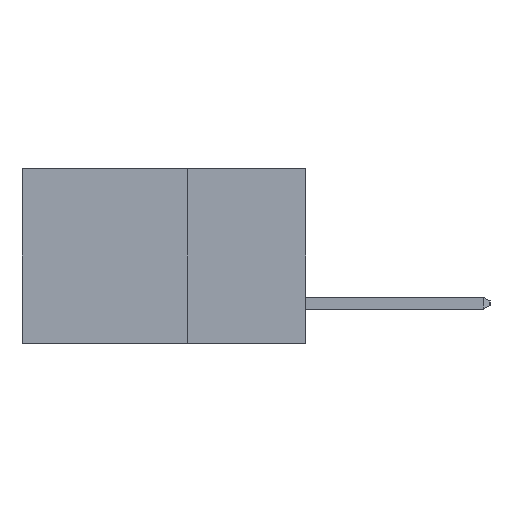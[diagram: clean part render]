
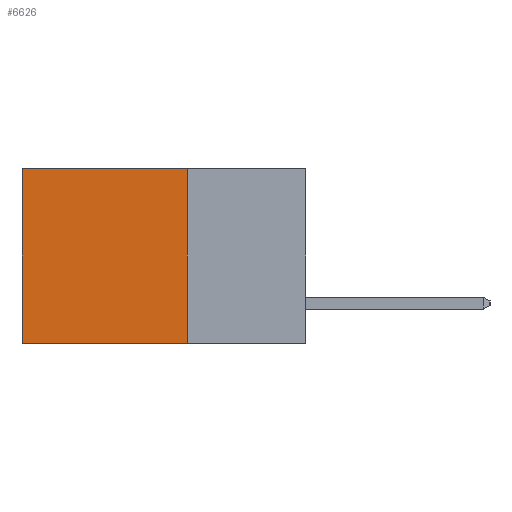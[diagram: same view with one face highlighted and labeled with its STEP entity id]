
A CAD part, left-side view. The second image highlights one B-rep face of the part: STEP entity #6626.
In plain terms, the highlighted planar face has unit normal (-1, 0, 0).
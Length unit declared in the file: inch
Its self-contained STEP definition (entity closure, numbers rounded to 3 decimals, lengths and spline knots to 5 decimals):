
#34 = CARTESIAN_POINT ( 'NONE',  ( 0.298, 0.25, 0. ) ) ;
#681 = VERTEX_POINT ( 'NONE', #8977 ) ;
#682 = EDGE_CURVE ( 'NONE', #681, #2729, #7356, .T. ) ;
#875 = CARTESIAN_POINT ( 'NONE',  ( 0.298, 0.25, 0. ) ) ;
#1124 = VECTOR ( 'NONE', #9426, 39.37008 ) ;
#1205 = DIRECTION ( 'NONE',  ( 0., 0., -1. ) ) ;
#1342 = LINE ( 'NONE', #8566, #5639 ) ;
#1620 = ORIENTED_EDGE ( 'NONE', *, *, #7671, .F. ) ;
#2339 = CARTESIAN_POINT ( 'NONE',  ( 0.298, 0.6, -0.37 ) ) ;
#2486 = VERTEX_POINT ( 'NONE', #10119 ) ;
#2727 = ORIENTED_EDGE ( 'NONE', *, *, #9683, .T. ) ;
#2729 = VERTEX_POINT ( 'NONE', #3269 ) ;
#2986 = EDGE_LOOP ( 'NONE', ( #2727, #3515, #1620, #4265 ) ) ;
#3269 = CARTESIAN_POINT ( 'NONE',  ( 0.298, 0.6, 0. ) ) ;
#3286 = LINE ( 'NONE', #7079, #1124 ) ;
#3515 = ORIENTED_EDGE ( 'NONE', *, *, #4010, .F. ) ;
#3601 = DIRECTION ( 'NONE',  ( 0., 1., 0. ) ) ;
#4010 = EDGE_CURVE ( 'NONE', #2486, #9549, #1342, .T. ) ;
#4142 = DIRECTION ( 'NONE',  ( 1., 0., 0. ) ) ;
#4265 = ORIENTED_EDGE ( 'NONE', *, *, #682, .T. ) ;
#4612 = DIRECTION ( 'NONE',  ( 0., 1., 0. ) ) ;
#5082 = FACE_OUTER_BOUND ( 'NONE', #2986, .T. ) ;
#5243 = VECTOR ( 'NONE', #3601, 39.37008 ) ;
#5244 = CARTESIAN_POINT ( 'NONE',  ( 0.298, 0.6, 0. ) ) ;
#5315 = LINE ( 'NONE', #5244, #9235 ) ;
#5639 = VECTOR ( 'NONE', #4612, 39.37008 ) ;
#6626 = ADVANCED_FACE ( 'NONE', ( #5082 ), #8906, .F. ) ;
#7079 = CARTESIAN_POINT ( 'NONE',  ( 0.298, 0.25, 0. ) ) ;
#7356 = LINE ( 'NONE', #34, #5243 ) ;
#7671 = EDGE_CURVE ( 'NONE', #681, #2486, #3286, .T. ) ;
#8566 = CARTESIAN_POINT ( 'NONE',  ( 0.298, 0.25, -0.37 ) ) ;
#8906 = PLANE ( 'NONE',  #9342 ) ;
#8977 = CARTESIAN_POINT ( 'NONE',  ( 0.298, 0.25, 0. ) ) ;
#9235 = VECTOR ( 'NONE', #1205, 39.37008 ) ;
#9342 = AXIS2_PLACEMENT_3D ( 'NONE', #875, #4142, #9653 ) ;
#9426 = DIRECTION ( 'NONE',  ( 0., 0., -1. ) ) ;
#9549 = VERTEX_POINT ( 'NONE', #2339 ) ;
#9653 = DIRECTION ( 'NONE',  ( 0., 0., -1. ) ) ;
#9683 = EDGE_CURVE ( 'NONE', #2729, #9549, #5315, .T. ) ;
#10119 = CARTESIAN_POINT ( 'NONE',  ( 0.298, 0.25, -0.37 ) ) ;
